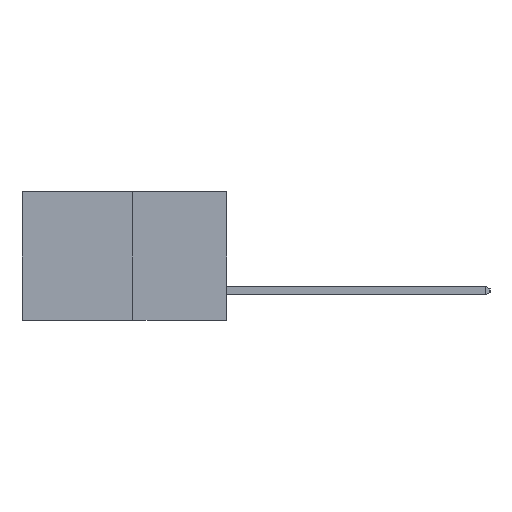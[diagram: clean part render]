
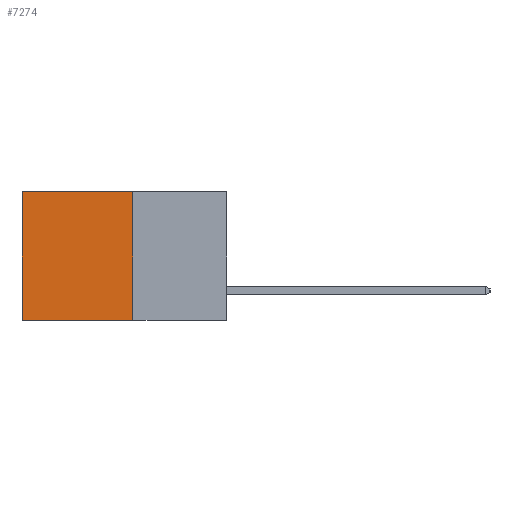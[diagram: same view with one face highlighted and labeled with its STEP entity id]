
A CAD part, left-side view. The second image highlights one B-rep face of the part: STEP entity #7274.
In plain terms, the highlighted planar face has unit normal (-1, 0, 0).
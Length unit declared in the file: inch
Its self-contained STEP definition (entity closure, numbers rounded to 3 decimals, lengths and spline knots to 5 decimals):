
#550 = ORIENTED_EDGE ( 'NONE', *, *, #8868, .T. ) ;
#965 = CARTESIAN_POINT ( 'NONE',  ( 0.277, 0.27, 0. ) ) ;
#4205 = VECTOR ( 'NONE', #5939, 39.37008 ) ;
#5166 = VECTOR ( 'NONE', #23866, 39.37008 ) ;
#5190 = DIRECTION ( 'NONE',  ( 1., 0., 0. ) ) ;
#5433 = EDGE_CURVE ( 'NONE', #11876, #9110, #10299, .T. ) ;
#5442 = ORIENTED_EDGE ( 'NONE', *, *, #10766, .F. ) ;
#5517 = CARTESIAN_POINT ( 'NONE',  ( 0.277, 0.59, -0.37 ) ) ;
#5939 = DIRECTION ( 'NONE',  ( 0., 1., 0. ) ) ;
#7274 = ADVANCED_FACE ( 'NONE', ( #13035 ), #17494, .F. ) ;
#8021 = EDGE_CURVE ( 'NONE', #22631, #9110, #15277, .T. ) ;
#8868 = EDGE_CURVE ( 'NONE', #11316, #22631, #9769, .T. ) ;
#9110 = VERTEX_POINT ( 'NONE', #24551 ) ;
#9717 = EDGE_LOOP ( 'NONE', ( #12032, #21876, #5442, #550 ) ) ;
#9769 = LINE ( 'NONE', #18462, #25221 ) ;
#10299 = LINE ( 'NONE', #20222, #4205 ) ;
#10375 = AXIS2_PLACEMENT_3D ( 'NONE', #23381, #5190, #19508 ) ;
#10766 = EDGE_CURVE ( 'NONE', #11316, #11876, #20807, .T. ) ;
#10939 = CARTESIAN_POINT ( 'NONE',  ( 0.277, 0.27, -0.37 ) ) ;
#11316 = VERTEX_POINT ( 'NONE', #965 ) ;
#11798 = CARTESIAN_POINT ( 'NONE',  ( 0.277, 0.27, -0.37 ) ) ;
#11876 = VERTEX_POINT ( 'NONE', #10939 ) ;
#12032 = ORIENTED_EDGE ( 'NONE', *, *, #8021, .T. ) ;
#13035 = FACE_OUTER_BOUND ( 'NONE', #9717, .T. ) ;
#13179 = CARTESIAN_POINT ( 'NONE',  ( 0.277, 0.59, 0. ) ) ;
#15277 = LINE ( 'NONE', #5517, #20656 ) ;
#17494 = PLANE ( 'NONE',  #10375 ) ;
#18462 = CARTESIAN_POINT ( 'NONE',  ( 0.277, 0.27, 0. ) ) ;
#19508 = DIRECTION ( 'NONE',  ( 0., 0., -1. ) ) ;
#19822 = DIRECTION ( 'NONE',  ( 0., 0., -1. ) ) ;
#20222 = CARTESIAN_POINT ( 'NONE',  ( 0.277, 0.27, -0.37 ) ) ;
#20468 = DIRECTION ( 'NONE',  ( 0., 1., 0. ) ) ;
#20656 = VECTOR ( 'NONE', #19822, 39.37008 ) ;
#20807 = LINE ( 'NONE', #11798, #5166 ) ;
#21876 = ORIENTED_EDGE ( 'NONE', *, *, #5433, .F. ) ;
#22631 = VERTEX_POINT ( 'NONE', #13179 ) ;
#23381 = CARTESIAN_POINT ( 'NONE',  ( 0.277, 0.27, -0.37 ) ) ;
#23866 = DIRECTION ( 'NONE',  ( 0., 0., -1. ) ) ;
#24551 = CARTESIAN_POINT ( 'NONE',  ( 0.277, 0.59, -0.37 ) ) ;
#25221 = VECTOR ( 'NONE', #20468, 39.37008 ) ;
